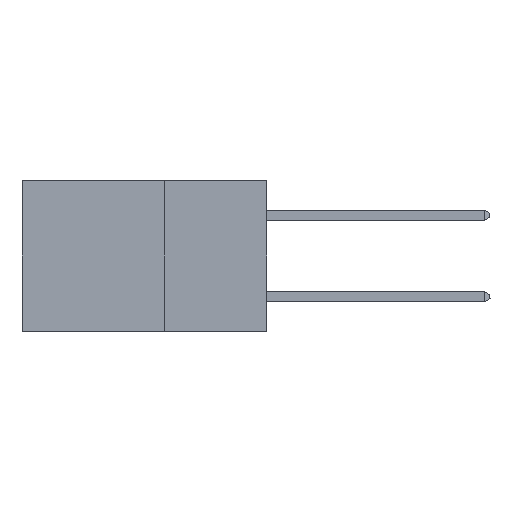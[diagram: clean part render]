
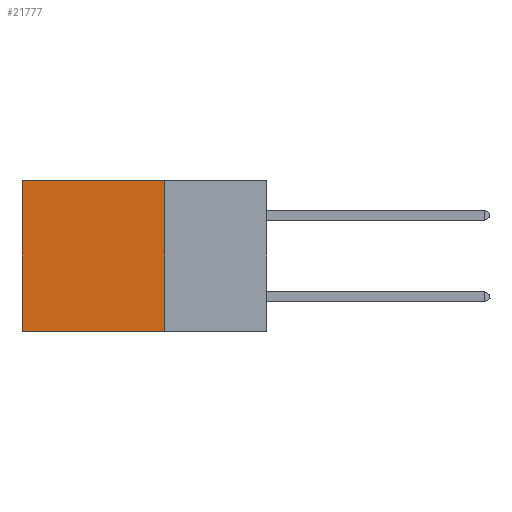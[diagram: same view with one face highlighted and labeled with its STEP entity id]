
A CAD part, left-side view. The second image highlights one B-rep face of the part: STEP entity #21777.
In plain terms, the highlighted planar face has unit normal (-1, 0, 0).
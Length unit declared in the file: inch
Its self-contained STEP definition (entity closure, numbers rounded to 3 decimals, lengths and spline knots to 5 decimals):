
#350 = VECTOR ( 'NONE', #4906, 39.37008 ) ;
#2939 = EDGE_CURVE ( 'NONE', #26913, #24702, #17122, .T. ) ;
#3963 = ORIENTED_EDGE ( 'NONE', *, *, #7479, .T. ) ;
#4906 = DIRECTION ( 'NONE',  ( 0., 1., 0. ) ) ;
#5564 = PLANE ( 'NONE',  #27453 ) ;
#6311 = FACE_OUTER_BOUND ( 'NONE', #13035, .T. ) ;
#6371 = VERTEX_POINT ( 'NONE', #18770 ) ;
#7199 = CARTESIAN_POINT ( 'NONE',  ( 0.2875, 0.25, -0.37 ) ) ;
#7311 = LINE ( 'NONE', #17335, #350 ) ;
#7479 = EDGE_CURVE ( 'NONE', #6371, #17320, #7311, .T. ) ;
#8501 = CARTESIAN_POINT ( 'NONE',  ( 0.2875, 0.25, 0. ) ) ;
#9232 = VECTOR ( 'NONE', #15698, 39.37008 ) ;
#10378 = DIRECTION ( 'NONE',  ( 0., 0., -1. ) ) ;
#10589 = VECTOR ( 'NONE', #22491, 39.37008 ) ;
#12619 = CARTESIAN_POINT ( 'NONE',  ( 0.2875, 0.6, 0. ) ) ;
#13035 = EDGE_LOOP ( 'NONE', ( #13261, #15099, #13330, #3963 ) ) ;
#13261 = ORIENTED_EDGE ( 'NONE', *, *, #29485, .T. ) ;
#13330 = ORIENTED_EDGE ( 'NONE', *, *, #15249, .F. ) ;
#15099 = ORIENTED_EDGE ( 'NONE', *, *, #2939, .F. ) ;
#15249 = EDGE_CURVE ( 'NONE', #6371, #26913, #26397, .T. ) ;
#15472 = CARTESIAN_POINT ( 'NONE',  ( 0.2875, 0.25, -0.37 ) ) ;
#15698 = DIRECTION ( 'NONE',  ( 0., 0., -1. ) ) ;
#17122 = LINE ( 'NONE', #7199, #10589 ) ;
#17320 = VERTEX_POINT ( 'NONE', #29125 ) ;
#17335 = CARTESIAN_POINT ( 'NONE',  ( 0.2875, 0.25, 0. ) ) ;
#17818 = CARTESIAN_POINT ( 'NONE',  ( 0.2875, 0.25, 0. ) ) ;
#18770 = CARTESIAN_POINT ( 'NONE',  ( 0.2875, 0.25, 0. ) ) ;
#21777 = ADVANCED_FACE ( 'NONE', ( #6311 ), #5564, .F. ) ;
#22095 = DIRECTION ( 'NONE',  ( 0., 0., -1. ) ) ;
#22445 = DIRECTION ( 'NONE',  ( 1., 0., 0. ) ) ;
#22491 = DIRECTION ( 'NONE',  ( 0., 1., 0. ) ) ;
#24702 = VERTEX_POINT ( 'NONE', #27031 ) ;
#26397 = LINE ( 'NONE', #8501, #9232 ) ;
#26913 = VERTEX_POINT ( 'NONE', #15472 ) ;
#27031 = CARTESIAN_POINT ( 'NONE',  ( 0.2875, 0.6, -0.37 ) ) ;
#27453 = AXIS2_PLACEMENT_3D ( 'NONE', #17818, #22445, #10378 ) ;
#27885 = LINE ( 'NONE', #12619, #30164 ) ;
#29125 = CARTESIAN_POINT ( 'NONE',  ( 0.2875, 0.6, 0. ) ) ;
#29485 = EDGE_CURVE ( 'NONE', #17320, #24702, #27885, .T. ) ;
#30164 = VECTOR ( 'NONE', #22095, 39.37008 ) ;
